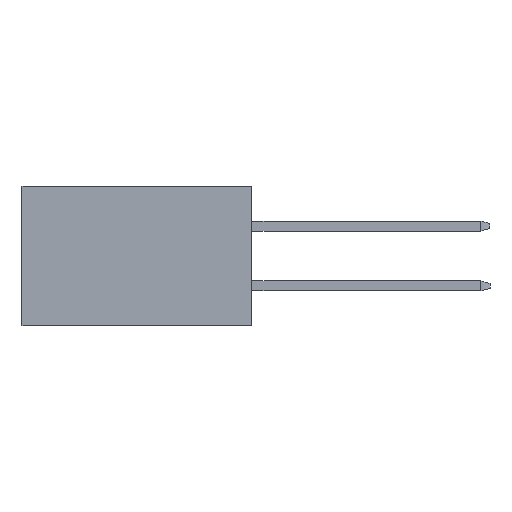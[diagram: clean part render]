
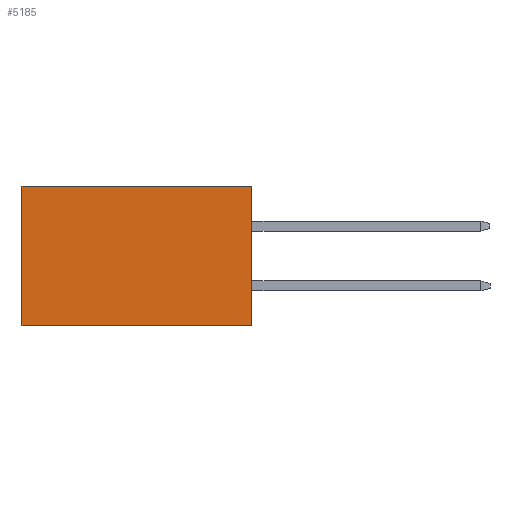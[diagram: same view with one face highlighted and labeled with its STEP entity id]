
A CAD part, left-side view. The second image highlights one B-rep face of the part: STEP entity #5185.
In plain terms, the highlighted planar face has unit normal (-1, 0, 0).
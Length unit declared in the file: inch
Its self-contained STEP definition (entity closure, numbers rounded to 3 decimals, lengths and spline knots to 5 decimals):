
#498 = LINE ( 'NONE', #10160, #7193 ) ;
#536 = EDGE_LOOP ( 'NONE', ( #10212, #16450, #5477, #5926 ) ) ;
#1968 = EDGE_CURVE ( 'NONE', #11359, #7205, #9662, .T. ) ;
#2421 = CARTESIAN_POINT ( 'NONE',  ( 0.3205, 0., -0.437 ) ) ;
#4124 = FACE_OUTER_BOUND ( 'NONE', #536, .T. ) ;
#4428 = EDGE_CURVE ( 'NONE', #4462, #11359, #498, .T. ) ;
#4462 = VERTEX_POINT ( 'NONE', #13224 ) ;
#4539 = AXIS2_PLACEMENT_3D ( 'NONE', #18138, #16747, #8238 ) ;
#4815 = DIRECTION ( 'NONE',  ( 0., 1., 0. ) ) ;
#5038 = DIRECTION ( 'NONE',  ( 0., 0., -1. ) ) ;
#5162 = VECTOR ( 'NONE', #5038, 39.37008 ) ;
#5185 = ADVANCED_FACE ( 'NONE', ( #4124 ), #12465, .F. ) ;
#5477 = ORIENTED_EDGE ( 'NONE', *, *, #5752, .F. ) ;
#5752 = EDGE_CURVE ( 'NONE', #4462, #11781, #12359, .T. ) ;
#5926 = ORIENTED_EDGE ( 'NONE', *, *, #4428, .T. ) ;
#6390 = DIRECTION ( 'NONE',  ( 0., 1., 0. ) ) ;
#7193 = VECTOR ( 'NONE', #4815, 39.37008 ) ;
#7205 = VERTEX_POINT ( 'NONE', #14314 ) ;
#7797 = LINE ( 'NONE', #13491, #12604 ) ;
#8193 = CARTESIAN_POINT ( 'NONE',  ( 0.3205, 0.72, 0. ) ) ;
#8238 = DIRECTION ( 'NONE',  ( 0., 0., -1. ) ) ;
#9662 = LINE ( 'NONE', #15424, #17487 ) ;
#10160 = CARTESIAN_POINT ( 'NONE',  ( 0.3205, 0., 0. ) ) ;
#10212 = ORIENTED_EDGE ( 'NONE', *, *, #1968, .T. ) ;
#11359 = VERTEX_POINT ( 'NONE', #8193 ) ;
#11781 = VERTEX_POINT ( 'NONE', #15801 ) ;
#12359 = LINE ( 'NONE', #2421, #5162 ) ;
#12465 = PLANE ( 'NONE',  #4539 ) ;
#12604 = VECTOR ( 'NONE', #6390, 39.37008 ) ;
#13224 = CARTESIAN_POINT ( 'NONE',  ( 0.3205, 0., 0. ) ) ;
#13491 = CARTESIAN_POINT ( 'NONE',  ( 0.3205, 0., -0.437 ) ) ;
#14314 = CARTESIAN_POINT ( 'NONE',  ( 0.3205, 0.72, -0.437 ) ) ;
#15337 = DIRECTION ( 'NONE',  ( 0., 0., -1. ) ) ;
#15424 = CARTESIAN_POINT ( 'NONE',  ( 0.3205, 0.72, -0.437 ) ) ;
#15801 = CARTESIAN_POINT ( 'NONE',  ( 0.3205, 0., -0.437 ) ) ;
#16406 = EDGE_CURVE ( 'NONE', #11781, #7205, #7797, .T. ) ;
#16450 = ORIENTED_EDGE ( 'NONE', *, *, #16406, .F. ) ;
#16747 = DIRECTION ( 'NONE',  ( 1., 0., 0. ) ) ;
#17487 = VECTOR ( 'NONE', #15337, 39.37008 ) ;
#18138 = CARTESIAN_POINT ( 'NONE',  ( 0.3205, 0., -0.437 ) ) ;
